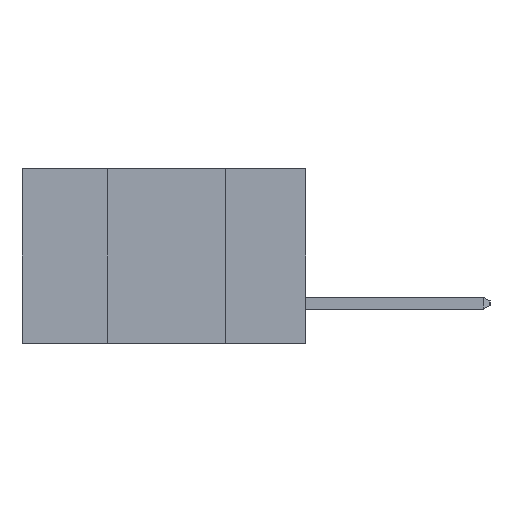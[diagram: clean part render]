
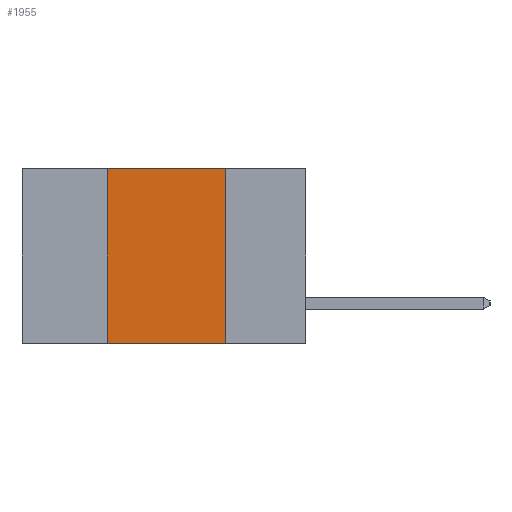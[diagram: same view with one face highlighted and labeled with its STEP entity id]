
A CAD part, left-side view. The second image highlights one B-rep face of the part: STEP entity #1955.
In plain terms, the highlighted planar face has unit normal (-1, 0, 0).
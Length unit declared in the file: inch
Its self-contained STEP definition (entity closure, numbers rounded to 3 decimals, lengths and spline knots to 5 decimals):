
#71 = CARTESIAN_POINT ( 'NONE',  ( 0., 0.42, 0. ) ) ;
#695 = VERTEX_POINT ( 'NONE', #19373 ) ;
#959 = ORIENTED_EDGE ( 'NONE', *, *, #10419, .F. ) ;
#1329 = VERTEX_POINT ( 'NONE', #71 ) ;
#1955 = ADVANCED_FACE ( 'NONE', ( #8325 ), #15619, .F. ) ;
#2094 = VECTOR ( 'NONE', #6215, 39.37008 ) ;
#2446 = VERTEX_POINT ( 'NONE', #4017 ) ;
#2690 = LINE ( 'NONE', #18047, #10374 ) ;
#2844 = VERTEX_POINT ( 'NONE', #15632 ) ;
#3900 = EDGE_CURVE ( 'NONE', #1329, #2446, #2690, .T. ) ;
#4017 = CARTESIAN_POINT ( 'NONE',  ( 0., 0.17, 0. ) ) ;
#4690 = CARTESIAN_POINT ( 'NONE',  ( 0., 0.17, -0.37 ) ) ;
#4827 = EDGE_LOOP ( 'NONE', ( #13223, #5121, #959, #15299 ) ) ;
#5121 = ORIENTED_EDGE ( 'NONE', *, *, #3900, .F. ) ;
#6215 = DIRECTION ( 'NONE',  ( 0., 0., -1. ) ) ;
#8048 = DIRECTION ( 'NONE',  ( 1., 0., 0. ) ) ;
#8325 = FACE_OUTER_BOUND ( 'NONE', #4827, .T. ) ;
#8674 = EDGE_CURVE ( 'NONE', #2446, #695, #13799, .T. ) ;
#9779 = EDGE_CURVE ( 'NONE', #2844, #695, #18280, .T. ) ;
#9828 = CARTESIAN_POINT ( 'NONE',  ( 0., 0.42, -0.37 ) ) ;
#9977 = CARTESIAN_POINT ( 'NONE',  ( 0., 0.6, -0.37 ) ) ;
#10374 = VECTOR ( 'NONE', #17846, 39.37008 ) ;
#10419 = EDGE_CURVE ( 'NONE', #2844, #1329, #12715, .T. ) ;
#10943 = VECTOR ( 'NONE', #11503, 39.37008 ) ;
#11503 = DIRECTION ( 'NONE',  ( 0., -1., 0. ) ) ;
#12244 = DIRECTION ( 'NONE',  ( 0., 0., -1. ) ) ;
#12461 = CARTESIAN_POINT ( 'NONE',  ( 0., 0.6, 0. ) ) ;
#12715 = LINE ( 'NONE', #9828, #16612 ) ;
#13223 = ORIENTED_EDGE ( 'NONE', *, *, #8674, .F. ) ;
#13799 = LINE ( 'NONE', #4690, #2094 ) ;
#15299 = ORIENTED_EDGE ( 'NONE', *, *, #9779, .T. ) ;
#15619 = PLANE ( 'NONE',  #17373 ) ;
#15632 = CARTESIAN_POINT ( 'NONE',  ( 0., 0.42, -0.37 ) ) ;
#16612 = VECTOR ( 'NONE', #18626, 39.37008 ) ;
#17373 = AXIS2_PLACEMENT_3D ( 'NONE', #12461, #8048, #12244 ) ;
#17846 = DIRECTION ( 'NONE',  ( 0., -1., 0. ) ) ;
#18047 = CARTESIAN_POINT ( 'NONE',  ( 0., 0.6, 0. ) ) ;
#18280 = LINE ( 'NONE', #9977, #10943 ) ;
#18626 = DIRECTION ( 'NONE',  ( 0., 0., 1. ) ) ;
#19373 = CARTESIAN_POINT ( 'NONE',  ( 0., 0.17, -0.37 ) ) ;
